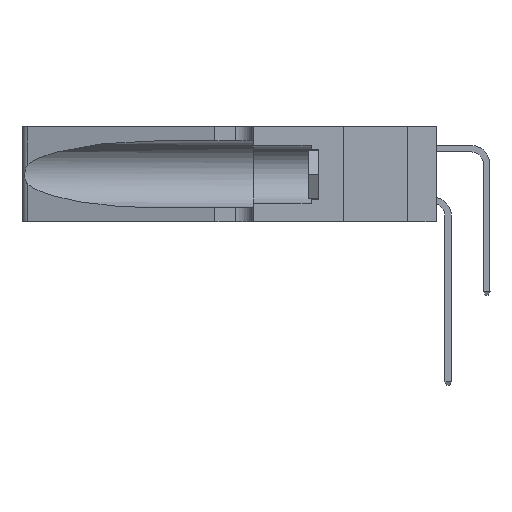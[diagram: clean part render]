
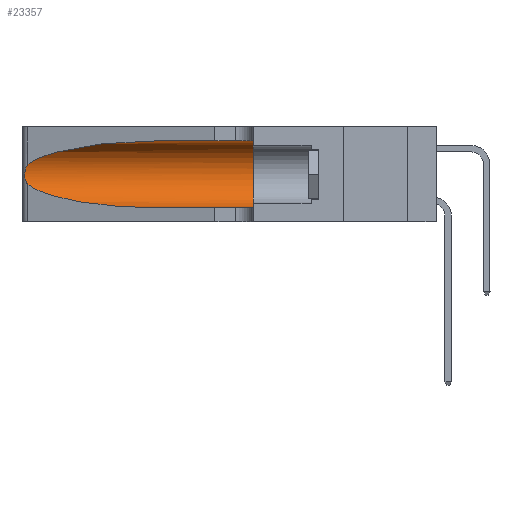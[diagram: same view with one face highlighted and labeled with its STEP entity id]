
A CAD part, left-side view. The second image highlights one B-rep face of the part: STEP entity #23357.
In plain terms, the highlighted cylindrical face has radius 3.308 mm (diameter 6.617 mm), a partial arc.
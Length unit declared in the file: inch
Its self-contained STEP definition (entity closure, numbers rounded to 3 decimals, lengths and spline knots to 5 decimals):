
#201 = CARTESIAN_POINT ( 'NONE',  ( 0.26018, 1.23835, 0.19895 ) ) ;
#578 = CARTESIAN_POINT ( 'NONE',  ( 0.25789, 1.23486, 0.15765 ) ) ;
#669 = CARTESIAN_POINT ( 'NONE',  ( 0.1305, 1.61858, 0.185 ) ) ;
#733 = CYLINDRICAL_SURFACE ( 'NONE', #17565, 0.13025 ) ;
#2255 = VERTEX_POINT ( 'NONE', #24051 ) ;
#3766 = VECTOR ( 'NONE', #4975, 39.37008 ) ;
#4975 = DIRECTION ( 'NONE',  ( 0., -1., 0. ) ) ;
#6915 = ORIENTED_EDGE ( 'NONE', *, *, #10606, .T. ) ;
#6966 = CARTESIAN_POINT ( 'NONE',  ( 0.25487, 1.22718, 0.22369 ) ) ;
#7098 = CARTESIAN_POINT ( 'NONE',  ( 0.25856, 1.23593, 0.16098 ) ) ;
#7411 = VERTEX_POINT ( 'NONE', #11725 ) ;
#7824 = LINE ( 'NONE', #17781, #3766 ) ;
#8663 = CARTESIAN_POINT ( 'NONE',  ( 0.2373, 1.15595, 0.28018 ) ) ;
#9092 = CARTESIAN_POINT ( 'NONE',  ( 0.1305, 0.72297, 0.31525 ) ) ;
#9160 = EDGE_CURVE ( 'NONE', #28858, #34302, #7824, .T. ) ;
#9240 = VERTEX_POINT ( 'NONE', #9092 ) ;
#9814 = DIRECTION ( 'NONE',  ( 0., 0., 1. ) ) ;
#9876 = CARTESIAN_POINT ( 'NONE',  ( 0.18966, 0.96281, 0.05475 ) ) ;
#10256 = CARTESIAN_POINT ( 'NONE',  ( 0.25787, 1.23484, 0.2124 ) ) ;
#10392 = CARTESIAN_POINT ( 'NONE',  ( 0.25487, 1.22718, 0.14631 ) ) ;
#10414 = FACE_OUTER_BOUND ( 'NONE', #22140, .T. ) ;
#10606 = EDGE_CURVE ( 'NONE', #9240, #7411, #12850, .T. ) ;
#11532 = ORIENTED_EDGE ( 'NONE', *, *, #30728, .F. ) ;
#11725 = CARTESIAN_POINT ( 'NONE',  ( 0.25487, 1.22718, 0.22369 ) ) ;
#11782 = CARTESIAN_POINT ( 'NONE',  ( 0.25487, 1.22718, 0.14631 ) ) ;
#12850 =( BOUNDED_CURVE ( )  B_SPLINE_CURVE ( 3, ( #18636, #18501, #8663, #14939 ),
 .UNSPECIFIED., .F., .T. ) 
 B_SPLINE_CURVE_WITH_KNOTS ( ( 4, 4 ),
 ( 1.5708, 2.84003 ),
 .UNSPECIFIED. ) 
 CURVE ( )  GEOMETRIC_REPRESENTATION_ITEM ( )  RATIONAL_B_SPLINE_CURVE ( ( 1., 0.87, 0.87, 1. ) ) 
 REPRESENTATION_ITEM ( '' )  );
#13530 = CARTESIAN_POINT ( 'NONE',  ( 0.26075, 1.23896, 0.178 ) ) ;
#13805 = CARTESIAN_POINT ( 'NONE',  ( 0.25639, 1.23186, 0.15144 ) ) ;
#14939 = CARTESIAN_POINT ( 'NONE',  ( 0.25487, 1.22718, 0.22369 ) ) ;
#15620 = EDGE_CURVE ( 'NONE', #9240, #2255, #30130, .T. ) ;
#15809 = CARTESIAN_POINT ( 'NONE',  ( 0.1305, 0.35, 0.185 ) ) ;
#16781 = CARTESIAN_POINT ( 'NONE',  ( 0.26017, 1.23833, 0.17102 ) ) ;
#17209 = B_SPLINE_CURVE_WITH_KNOTS ( 'NONE', 3,
 ( #6966, #33333, #29774, #10256, #23081, #201, #33078, #13530, #16781, #7098, #578, #13805, #29909, #10392 ),
 .UNSPECIFIED., .F., .F.,
 ( 4, 2, 2, 2, 2, 2, 4 ),
 ( 0., 0.00027, 0.00053, 0.00107, 0.0016, 0.00187, 0.00214 ),
 .UNSPECIFIED. ) ;
#17565 = AXIS2_PLACEMENT_3D ( 'NONE', #669, #39713, #20190 ) ;
#17781 = CARTESIAN_POINT ( 'NONE',  ( 0.1305, 1.61858, 0.05475 ) ) ;
#18301 = CARTESIAN_POINT ( 'NONE',  ( 0.2373, 1.15595, 0.08982 ) ) ;
#18501 = CARTESIAN_POINT ( 'NONE',  ( 0.18966, 0.96281, 0.31525 ) ) ;
#18636 = CARTESIAN_POINT ( 'NONE',  ( 0.1305, 0.72297, 0.31525 ) ) ;
#18966 = ORIENTED_EDGE ( 'NONE', *, *, #27180, .T. ) ;
#20190 = DIRECTION ( 'NONE',  ( 0., 0., -1. ) ) ;
#21339 = AXIS2_PLACEMENT_3D ( 'NONE', #15809, #39034, #9814 ) ;
#22140 = EDGE_LOOP ( 'NONE', ( #6915, #40219, #18966, #29359, #11532, #29782 ) ) ;
#22194 = CARTESIAN_POINT ( 'NONE',  ( 0.1305, 0.35, 0.05475 ) ) ;
#22956 = VERTEX_POINT ( 'NONE', #24679 ) ;
#23081 = CARTESIAN_POINT ( 'NONE',  ( 0.25854, 1.2359, 0.20912 ) ) ;
#23357 = ADVANCED_FACE ( 'NONE', ( #10414 ), #733, .F. ) ;
#24051 = CARTESIAN_POINT ( 'NONE',  ( 0.1305, 0.35, 0.31525 ) ) ;
#24679 = CARTESIAN_POINT ( 'NONE',  ( 0.25487, 1.22718, 0.14631 ) ) ;
#26105 = CARTESIAN_POINT ( 'NONE',  ( 0.1305, 0.72297, 0.05475 ) ) ;
#27180 = EDGE_CURVE ( 'NONE', #22956, #28858, #31147, .T. ) ;
#28858 = VERTEX_POINT ( 'NONE', #26105 ) ;
#29359 = ORIENTED_EDGE ( 'NONE', *, *, #9160, .T. ) ;
#29577 = VECTOR ( 'NONE', #31047, 39.37008 ) ;
#29774 = CARTESIAN_POINT ( 'NONE',  ( 0.25639, 1.23184, 0.21858 ) ) ;
#29782 = ORIENTED_EDGE ( 'NONE', *, *, #15620, .F. ) ;
#29909 = CARTESIAN_POINT ( 'NONE',  ( 0.25555, 1.22993, 0.14849 ) ) ;
#30130 = LINE ( 'NONE', #30756, #29577 ) ;
#30728 = EDGE_CURVE ( 'NONE', #2255, #34302, #35084, .T. ) ;
#30756 = CARTESIAN_POINT ( 'NONE',  ( 0.1305, 1.61858, 0.31525 ) ) ;
#31047 = DIRECTION ( 'NONE',  ( 0., -1., 0. ) ) ;
#31147 =( BOUNDED_CURVE ( )  B_SPLINE_CURVE ( 3, ( #11782, #18301, #9876, #39093 ),
 .UNSPECIFIED., .F., .F. ) 
 B_SPLINE_CURVE_WITH_KNOTS ( ( 4, 4 ),
 ( 3.44316, 4.71239 ),
 .UNSPECIFIED. ) 
 CURVE ( )  GEOMETRIC_REPRESENTATION_ITEM ( )  RATIONAL_B_SPLINE_CURVE ( ( 1., 0.87, 0.87, 1. ) ) 
 REPRESENTATION_ITEM ( '' )  );
#33078 = CARTESIAN_POINT ( 'NONE',  ( 0.26075, 1.23896, 0.19203 ) ) ;
#33333 = CARTESIAN_POINT ( 'NONE',  ( 0.25555, 1.22994, 0.2215 ) ) ;
#34302 = VERTEX_POINT ( 'NONE', #22194 ) ;
#35084 = CIRCLE ( 'NONE', #21339, 0.13025 ) ;
#36393 = EDGE_CURVE ( 'NONE', #7411, #22956, #17209, .T. ) ;
#39034 = DIRECTION ( 'NONE',  ( 0., 1., 0. ) ) ;
#39093 = CARTESIAN_POINT ( 'NONE',  ( 0.1305, 0.72297, 0.05475 ) ) ;
#39713 = DIRECTION ( 'NONE',  ( 0., -1., 0. ) ) ;
#40219 = ORIENTED_EDGE ( 'NONE', *, *, #36393, .T. ) ;
